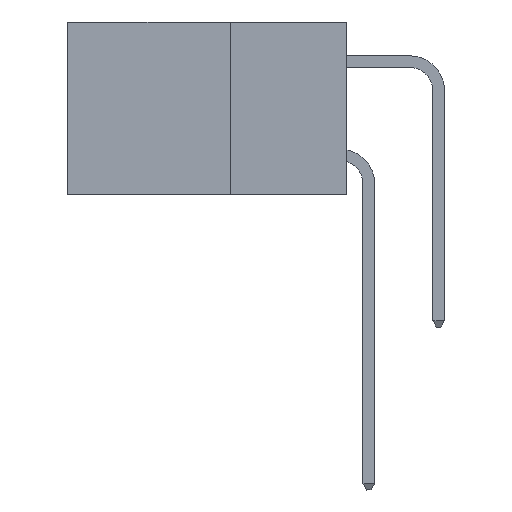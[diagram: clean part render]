
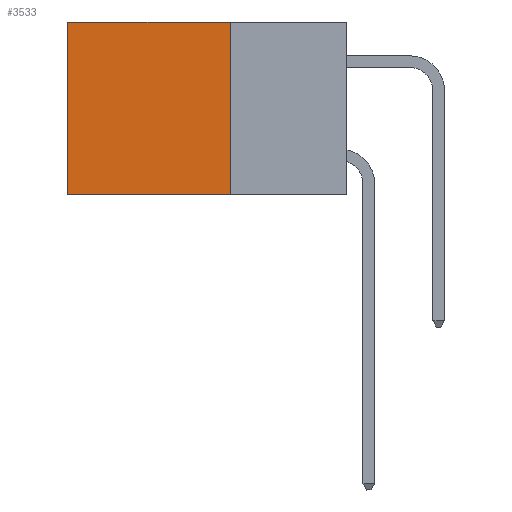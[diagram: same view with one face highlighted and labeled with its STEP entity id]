
A CAD part, left-side view. The second image highlights one B-rep face of the part: STEP entity #3533.
In plain terms, the highlighted planar face has unit normal (-1, 0, 0).
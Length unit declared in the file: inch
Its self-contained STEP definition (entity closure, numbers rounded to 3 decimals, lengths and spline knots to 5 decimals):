
#478 = CARTESIAN_POINT ( 'NONE',  ( 0.2875, 0.25, -0.37 ) ) ;
#2094 = CARTESIAN_POINT ( 'NONE',  ( 0.2875, 0.25, 0. ) ) ;
#2440 = VERTEX_POINT ( 'NONE', #28928 ) ;
#3533 = ADVANCED_FACE ( 'NONE', ( #19553 ), #11234, .F. ) ;
#4112 = VECTOR ( 'NONE', #6870, 39.37008 ) ;
#5272 = DIRECTION ( 'NONE',  ( 0., 1., 0. ) ) ;
#5795 = EDGE_CURVE ( 'NONE', #22233, #2440, #6162, .T. ) ;
#6162 = LINE ( 'NONE', #2094, #19546 ) ;
#6182 = AXIS2_PLACEMENT_3D ( 'NONE', #26106, #13375, #6993 ) ;
#6690 = LINE ( 'NONE', #16246, #4112 ) ;
#6870 = DIRECTION ( 'NONE',  ( 0., 0., -1. ) ) ;
#6993 = DIRECTION ( 'NONE',  ( 0., 0., -1. ) ) ;
#9227 = VECTOR ( 'NONE', #15014, 39.37008 ) ;
#9610 = VECTOR ( 'NONE', #5272, 39.37008 ) ;
#10270 = CARTESIAN_POINT ( 'NONE',  ( 0.2875, 0.25, 0. ) ) ;
#10760 = ORIENTED_EDGE ( 'NONE', *, *, #27549, .F. ) ;
#10785 = VERTEX_POINT ( 'NONE', #15088 ) ;
#11234 = PLANE ( 'NONE',  #6182 ) ;
#13172 = EDGE_CURVE ( 'NONE', #14971, #10785, #29250, .T. ) ;
#13375 = DIRECTION ( 'NONE',  ( 1., 0., 0. ) ) ;
#13405 = EDGE_LOOP ( 'NONE', ( #25091, #28856, #10760, #18689 ) ) ;
#14971 = VERTEX_POINT ( 'NONE', #16762 ) ;
#15014 = DIRECTION ( 'NONE',  ( 0., 0., -1. ) ) ;
#15088 = CARTESIAN_POINT ( 'NONE',  ( 0.2875, 0.6, -0.37 ) ) ;
#16246 = CARTESIAN_POINT ( 'NONE',  ( 0.2875, 0.6, 0. ) ) ;
#16762 = CARTESIAN_POINT ( 'NONE',  ( 0.2875, 0.25, -0.37 ) ) ;
#18689 = ORIENTED_EDGE ( 'NONE', *, *, #5795, .T. ) ;
#19546 = VECTOR ( 'NONE', #22583, 39.37008 ) ;
#19553 = FACE_OUTER_BOUND ( 'NONE', #13405, .T. ) ;
#22233 = VERTEX_POINT ( 'NONE', #26744 ) ;
#22583 = DIRECTION ( 'NONE',  ( 0., 1., 0. ) ) ;
#25091 = ORIENTED_EDGE ( 'NONE', *, *, #27857, .T. ) ;
#25568 = LINE ( 'NONE', #10270, #9227 ) ;
#26106 = CARTESIAN_POINT ( 'NONE',  ( 0.2875, 0.25, 0. ) ) ;
#26744 = CARTESIAN_POINT ( 'NONE',  ( 0.2875, 0.25, 0. ) ) ;
#27549 = EDGE_CURVE ( 'NONE', #22233, #14971, #25568, .T. ) ;
#27857 = EDGE_CURVE ( 'NONE', #2440, #10785, #6690, .T. ) ;
#28856 = ORIENTED_EDGE ( 'NONE', *, *, #13172, .F. ) ;
#28928 = CARTESIAN_POINT ( 'NONE',  ( 0.2875, 0.6, 0. ) ) ;
#29250 = LINE ( 'NONE', #478, #9610 ) ;
